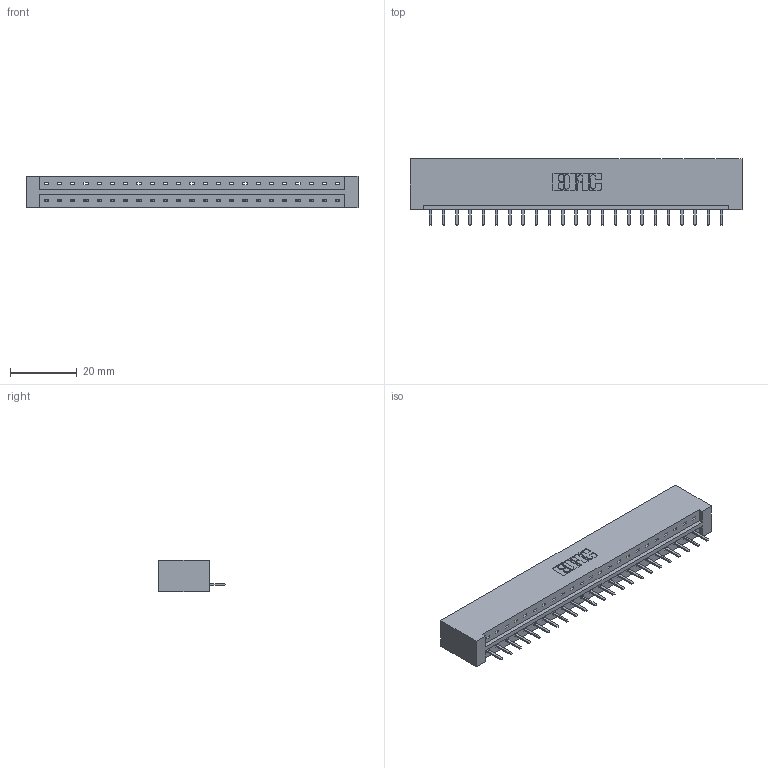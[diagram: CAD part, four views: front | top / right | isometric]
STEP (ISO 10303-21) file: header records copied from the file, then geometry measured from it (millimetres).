
FILE_DESCRIPTION (( 'STEP AP203' ), '1' );
FILE_NAME ('333-023-520-101.STEP', '2018-08-02T03:10:13', ( '' ), ( '' ), 'SwSTEP 2.0', 'SolidWorks 2016', '' );
FILE_SCHEMA (( 'CONFIG_CONTROL_DESIGN' ));
Length unit declared in the file: inch
Products named in the file (3): 333 Part_Lugless; 345-292-001_345-293-120; 333-023-520-101
Assembly tree (24 placements, depth 2):
  333-023-520-101
    333 Part_Lugless
    345-292-001_345-293-120  x23
Bounding box: 99.39 x 20.02 x 9.4 mm (x, y, z)
Volume: 10384.6 mm3; surface area: 10836.1 mm2
Topology: 24 solids, 24 shells, 1532 faces, 4519 edges, 2950 vertices
Faces by surface type: plane 1078, cylinder 454
Entity records: 16355 total; most frequent: CARTESIAN_POINT 2843, ORIENTED_EDGE 2790, DIRECTION 2417, EDGE_CURVE 1395, LINE 1271, VECTOR 1271, VERTEX_POINT 926, AXIS2_PLACEMENT_3D 573
